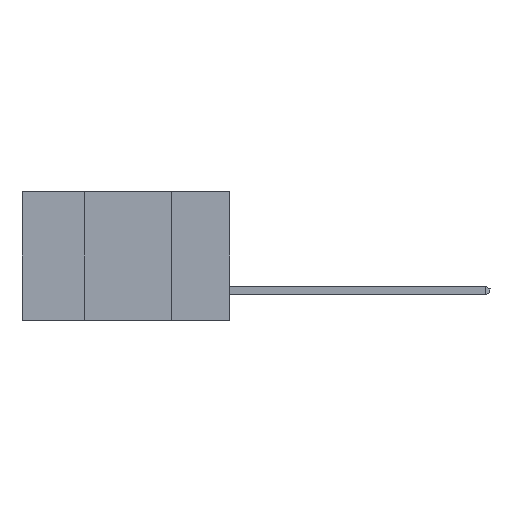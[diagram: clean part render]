
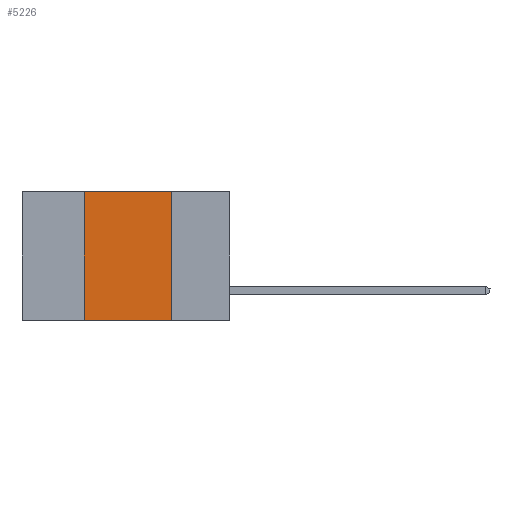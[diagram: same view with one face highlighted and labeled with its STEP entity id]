
A CAD part, left-side view. The second image highlights one B-rep face of the part: STEP entity #5226.
In plain terms, the highlighted planar face has unit normal (-1, 0, 0).
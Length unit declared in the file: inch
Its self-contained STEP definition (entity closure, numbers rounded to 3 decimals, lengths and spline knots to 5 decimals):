
#1250 = VERTEX_POINT ( 'NONE', #7973 ) ;
#1529 = DIRECTION ( 'NONE',  ( 0., 0., -1. ) ) ;
#2574 = EDGE_CURVE ( 'NONE', #12832, #22541, #4857, .T. ) ;
#3034 = CARTESIAN_POINT ( 'NONE',  ( 0., 0.6, 0. ) ) ;
#3166 = CARTESIAN_POINT ( 'NONE',  ( 0., 0.42, -0.37 ) ) ;
#3322 = DIRECTION ( 'NONE',  ( 0., 0., -1. ) ) ;
#4857 = LINE ( 'NONE', #18974, #19136 ) ;
#5226 = ADVANCED_FACE ( 'NONE', ( #20777 ), #13178, .F. ) ;
#5502 = ORIENTED_EDGE ( 'NONE', *, *, #19359, .F. ) ;
#6128 = EDGE_LOOP ( 'NONE', ( #7871, #5502, #8461, #22754 ) ) ;
#7871 = ORIENTED_EDGE ( 'NONE', *, *, #16383, .F. ) ;
#7973 = CARTESIAN_POINT ( 'NONE',  ( 0., 0.42, 0. ) ) ;
#8461 = ORIENTED_EDGE ( 'NONE', *, *, #11950, .F. ) ;
#8512 = CARTESIAN_POINT ( 'NONE',  ( 0., 0.17, 0. ) ) ;
#8630 = DIRECTION ( 'NONE',  ( 1., 0., 0. ) ) ;
#8940 = LINE ( 'NONE', #3034, #10865 ) ;
#10267 = VECTOR ( 'NONE', #13091, 39.37008 ) ;
#10865 = VECTOR ( 'NONE', #24240, 39.37008 ) ;
#11950 = EDGE_CURVE ( 'NONE', #12832, #1250, #13473, .T. ) ;
#12832 = VERTEX_POINT ( 'NONE', #3166 ) ;
#13091 = DIRECTION ( 'NONE',  ( 0., 0., 1. ) ) ;
#13178 = PLANE ( 'NONE',  #21645 ) ;
#13473 = LINE ( 'NONE', #21325, #10267 ) ;
#13526 = VERTEX_POINT ( 'NONE', #8512 ) ;
#15272 = LINE ( 'NONE', #18998, #20631 ) ;
#16383 = EDGE_CURVE ( 'NONE', #13526, #22541, #15272, .T. ) ;
#17202 = CARTESIAN_POINT ( 'NONE',  ( 0., 0.6, 0. ) ) ;
#18480 = DIRECTION ( 'NONE',  ( 0., -1., 0. ) ) ;
#18974 = CARTESIAN_POINT ( 'NONE',  ( 0., 0.6, -0.37 ) ) ;
#18998 = CARTESIAN_POINT ( 'NONE',  ( 0., 0.17, -0.37 ) ) ;
#19136 = VECTOR ( 'NONE', #18480, 39.37008 ) ;
#19359 = EDGE_CURVE ( 'NONE', #1250, #13526, #8940, .T. ) ;
#19592 = CARTESIAN_POINT ( 'NONE',  ( 0., 0.17, -0.37 ) ) ;
#20631 = VECTOR ( 'NONE', #1529, 39.37008 ) ;
#20777 = FACE_OUTER_BOUND ( 'NONE', #6128, .T. ) ;
#21325 = CARTESIAN_POINT ( 'NONE',  ( 0., 0.42, -0.37 ) ) ;
#21645 = AXIS2_PLACEMENT_3D ( 'NONE', #17202, #8630, #3322 ) ;
#22541 = VERTEX_POINT ( 'NONE', #19592 ) ;
#22754 = ORIENTED_EDGE ( 'NONE', *, *, #2574, .T. ) ;
#24240 = DIRECTION ( 'NONE',  ( 0., -1., 0. ) ) ;
